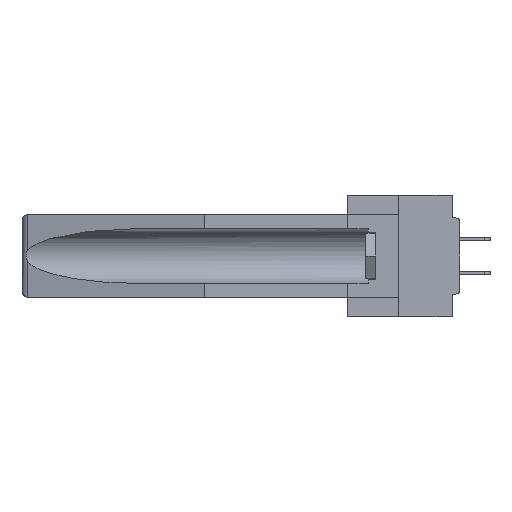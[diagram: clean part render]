
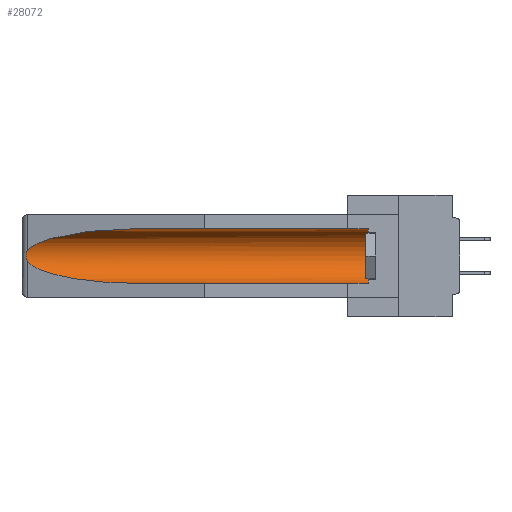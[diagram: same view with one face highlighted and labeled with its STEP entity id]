
A CAD part, left-side view. The second image highlights one B-rep face of the part: STEP entity #28072.
In plain terms, the highlighted cylindrical face has radius 2.857 mm (diameter 5.715 mm), a partial arc.
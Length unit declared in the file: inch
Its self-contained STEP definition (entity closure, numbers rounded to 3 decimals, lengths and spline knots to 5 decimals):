
#1205 = EDGE_LOOP ( 'NONE', ( #26374, #24103, #11946, #5892, #6483, #16915 ) ) ;
#1250 = CARTESIAN_POINT ( 'NONE',  ( 0.26537, 1.52718, -0.14972 ) ) ;
#1351 = CARTESIAN_POINT ( 'NONE',  ( 0.26537, 1.52718, -0.19328 ) ) ;
#2771 = AXIS2_PLACEMENT_3D ( 'NONE', #21606, #21086, #6244 ) ;
#5454 = CARTESIAN_POINT ( 'NONE',  ( 0.25451, 1.48313, -0.09465 ) ) ;
#5892 = ORIENTED_EDGE ( 'NONE', *, *, #14414, .F. ) ;
#6244 = DIRECTION ( 'NONE',  ( 0., 0., 1. ) ) ;
#6461 = EDGE_CURVE ( 'NONE', #16501, #19933, #40144, .T. ) ;
#6483 = ORIENTED_EDGE ( 'NONE', *, *, #21885, .T. ) ;
#9754 = CARTESIAN_POINT ( 'NONE',  ( 0.26597, 1.52961, -0.15275 ) ) ;
#9802 = VERTEX_POINT ( 'NONE', #1250 ) ;
#9882 = CARTESIAN_POINT ( 'NONE',  ( 0.2673, 1.5327, -0.16383 ) ) ;
#10536 = CARTESIAN_POINT ( 'NONE',  ( 0.155, 0.126, -0.1715 ) ) ;
#10637 = VERTEX_POINT ( 'NONE', #23117 ) ;
#10664 = DIRECTION ( 'NONE',  ( 0., 0., 1. ) ) ;
#10751 = CARTESIAN_POINT ( 'NONE',  ( 0.25451, 1.48313, -0.24835 ) ) ;
#11686 = CARTESIAN_POINT ( 'NONE',  ( 0.155, 1.07973, -0.284 ) ) ;
#11946 = ORIENTED_EDGE ( 'NONE', *, *, #39076, .T. ) ;
#12922 = CARTESIAN_POINT ( 'NONE',  ( 0.26537, 1.52718, -0.14972 ) ) ;
#13009 =( BOUNDED_CURVE ( )  B_SPLINE_CURVE ( 3, ( #23398, #10751, #30547, #37088 ),
 .UNSPECIFIED., .F., .T. ) 
 B_SPLINE_CURVE_WITH_KNOTS ( ( 4, 4 ),
 ( 0.1948, 1.5708 ),
 .UNSPECIFIED. ) 
 CURVE ( )  GEOMETRIC_REPRESENTATION_ITEM ( )  RATIONAL_B_SPLINE_CURVE ( ( 1., 0.848, 0.848, 1. ) ) 
 REPRESENTATION_ITEM ( '' )  );
#13523 =( BOUNDED_CURVE ( )  B_SPLINE_CURVE ( 3, ( #34125, #40618, #5454, #38128 ),
 .UNSPECIFIED., .F., .T. ) 
 B_SPLINE_CURVE_WITH_KNOTS ( ( 4, 4 ),
 ( 4.71239, 6.08839 ),
 .UNSPECIFIED. ) 
 CURVE ( )  GEOMETRIC_REPRESENTATION_ITEM ( )  RATIONAL_B_SPLINE_CURVE ( ( 1., 0.848, 0.848, 1. ) ) 
 REPRESENTATION_ITEM ( '' )  );
#14414 = EDGE_CURVE ( 'NONE', #10637, #39574, #39441, .T. ) ;
#14436 = CARTESIAN_POINT ( 'NONE',  ( 0.26537, 1.52718, -0.19328 ) ) ;
#15226 = VERTEX_POINT ( 'NONE', #1351 ) ;
#15664 = CARTESIAN_POINT ( 'NONE',  ( 0.155, -0.30754, -0.284 ) ) ;
#16228 = CARTESIAN_POINT ( 'NONE',  ( 0.2675, 1.53308, -0.17534 ) ) ;
#16501 = VERTEX_POINT ( 'NONE', #26110 ) ;
#16915 = ORIENTED_EDGE ( 'NONE', *, *, #6461, .T. ) ;
#19295 = CARTESIAN_POINT ( 'NONE',  ( 0.26654, 1.53092, -0.15636 ) ) ;
#19431 = CARTESIAN_POINT ( 'NONE',  ( 0.2673, 1.53269, -0.17917 ) ) ;
#19933 = VERTEX_POINT ( 'NONE', #22191 ) ;
#21025 = AXIS2_PLACEMENT_3D ( 'NONE', #10536, #29619, #10664 ) ;
#21086 = DIRECTION ( 'NONE',  ( 0., 1., 0. ) ) ;
#21606 = CARTESIAN_POINT ( 'NONE',  ( 0.155, -0.30754, -0.1715 ) ) ;
#21885 = EDGE_CURVE ( 'NONE', #10637, #16501, #35097, .T. ) ;
#22191 = CARTESIAN_POINT ( 'NONE',  ( 0.155, 1.07973, -0.059 ) ) ;
#22640 = CARTESIAN_POINT ( 'NONE',  ( 0.26655, 1.53094, -0.18657 ) ) ;
#22981 = EDGE_CURVE ( 'NONE', #9802, #15226, #39929, .T. ) ;
#23117 = CARTESIAN_POINT ( 'NONE',  ( 0.155, 0.126, -0.284 ) ) ;
#23398 = CARTESIAN_POINT ( 'NONE',  ( 0.26537, 1.52718, -0.19328 ) ) ;
#24103 = ORIENTED_EDGE ( 'NONE', *, *, #22981, .T. ) ;
#26110 = CARTESIAN_POINT ( 'NONE',  ( 0.155, 0.126, -0.059 ) ) ;
#26374 = ORIENTED_EDGE ( 'NONE', *, *, #30760, .T. ) ;
#27523 = CARTESIAN_POINT ( 'NONE',  ( 0.155, -0.30754, -0.059 ) ) ;
#28072 = ADVANCED_FACE ( 'NONE', ( #29104 ), #32105, .F. ) ;
#28692 = CARTESIAN_POINT ( 'NONE',  ( 0.2675, 1.53308, -0.16763 ) ) ;
#29104 = FACE_OUTER_BOUND ( 'NONE', #1205, .T. ) ;
#29528 = VECTOR ( 'NONE', #31718, 39.37008 ) ;
#29619 = DIRECTION ( 'NONE',  ( 0., -1., 0. ) ) ;
#29908 = CARTESIAN_POINT ( 'NONE',  ( 0.26597, 1.5296, -0.19026 ) ) ;
#30547 = CARTESIAN_POINT ( 'NONE',  ( 0.21114, 1.30732, -0.284 ) ) ;
#30760 = EDGE_CURVE ( 'NONE', #19933, #9802, #13523, .T. ) ;
#31718 = DIRECTION ( 'NONE',  ( 0., 1., 0. ) ) ;
#32105 = CYLINDRICAL_SURFACE ( 'NONE', #2771, 0.1125 ) ;
#34125 = CARTESIAN_POINT ( 'NONE',  ( 0.155, 1.07973, -0.059 ) ) ;
#35097 = CIRCLE ( 'NONE', #21025, 0.1125 ) ;
#36190 = VECTOR ( 'NONE', #37625, 39.37008 ) ;
#37088 = CARTESIAN_POINT ( 'NONE',  ( 0.155, 1.07973, -0.284 ) ) ;
#37625 = DIRECTION ( 'NONE',  ( 0., 1., 0. ) ) ;
#38128 = CARTESIAN_POINT ( 'NONE',  ( 0.26537, 1.52718, -0.14972 ) ) ;
#39076 = EDGE_CURVE ( 'NONE', #15226, #39574, #13009, .T. ) ;
#39441 = LINE ( 'NONE', #15664, #29528 ) ;
#39574 = VERTEX_POINT ( 'NONE', #11686 ) ;
#39929 = B_SPLINE_CURVE_WITH_KNOTS ( 'NONE', 3,
 ( #12922, #9754, #19295, #9882, #28692, #16228, #19431, #22640, #29908, #14436 ),
 .UNSPECIFIED., .F., .F.,
 ( 4, 2, 2, 2, 4 ),
 ( 0., 0.00029, 0.00058, 0.00087, 0.00117 ),
 .UNSPECIFIED. ) ;
#40144 = LINE ( 'NONE', #27523, #36190 ) ;
#40618 = CARTESIAN_POINT ( 'NONE',  ( 0.21114, 1.30732, -0.059 ) ) ;
